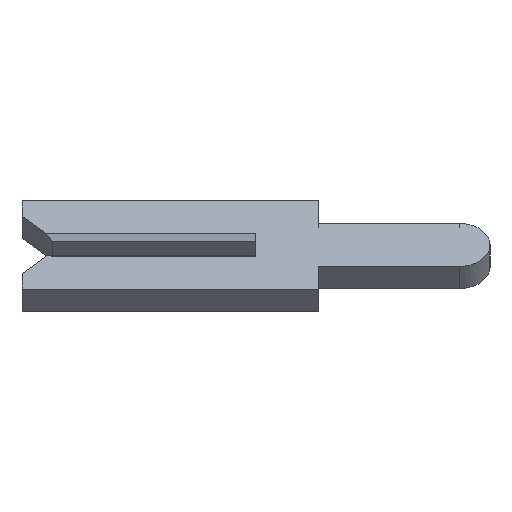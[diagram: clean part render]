
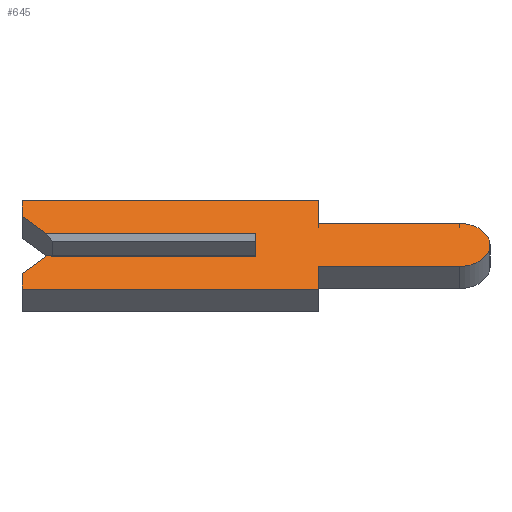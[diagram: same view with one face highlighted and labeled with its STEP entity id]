
A CAD part, left-side view. The second image highlights one B-rep face of the part: STEP entity #645.
In plain terms, the highlighted face is planar.
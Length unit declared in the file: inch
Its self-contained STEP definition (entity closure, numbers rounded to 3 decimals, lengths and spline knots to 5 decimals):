
#2 = VERTEX_POINT ( 'NONE', #682 ) ;
#9 = VERTEX_POINT ( 'NONE', #167 ) ;
#14 = VECTOR ( 'NONE', #315, 39.37008 ) ;
#22 = DIRECTION ( 'NONE',  ( 0., -1., 0. ) ) ;
#23 = ORIENTED_EDGE ( 'NONE', *, *, #552, .F. ) ;
#30 = CARTESIAN_POINT ( 'NONE',  ( -0.01, -0.04, 0.04 ) ) ;
#38 = ORIENTED_EDGE ( 'NONE', *, *, #473, .F. ) ;
#52 = CARTESIAN_POINT ( 'NONE',  ( -0.01, 0.15, -0.026 ) ) ;
#77 = FACE_OUTER_BOUND ( 'NONE', #510, .T. ) ;
#93 = EDGE_CURVE ( 'NONE', #1032, #974, #1175, .T. ) ;
#94 = LINE ( 'NONE', #275, #698 ) ;
#96 = ORIENTED_EDGE ( 'NONE', *, *, #981, .F. ) ;
#99 = EDGE_CURVE ( 'NONE', #467, #673, #94, .T. ) ;
#143 = ORIENTED_EDGE ( 'NONE', *, *, #973, .F. ) ;
#149 = VECTOR ( 'NONE', #853, 39.37008 ) ;
#152 = CARTESIAN_POINT ( 'NONE',  ( -0.01, -0.1305, 0.0195 ) ) ;
#167 = CARTESIAN_POINT ( 'NONE',  ( -0.01, 0.15, 0.04 ) ) ;
#171 = ORIENTED_EDGE ( 'NONE', *, *, #1260, .F. ) ;
#174 = DIRECTION ( 'NONE',  ( 0., 1., 0. ) ) ;
#180 = CARTESIAN_POINT ( 'NONE',  ( -0.01, 0., -0.01 ) ) ;
#188 = CARTESIAN_POINT ( 'NONE',  ( -0.01, 0.15, 0.026 ) ) ;
#198 = ORIENTED_EDGE ( 'NONE', *, *, #1116, .F. ) ;
#201 = AXIS2_PLACEMENT_3D ( 'NONE', #718, #932, #1027 ) ;
#202 = LINE ( 'NONE', #454, #268 ) ;
#247 = VERTEX_POINT ( 'NONE', #1136 ) ;
#257 = CARTESIAN_POINT ( 'NONE',  ( -0.01, 0.15, 0.01 ) ) ;
#263 = ORIENTED_EDGE ( 'NONE', *, *, #450, .F. ) ;
#266 = LINE ( 'NONE', #834, #333 ) ;
#268 = VECTOR ( 'NONE', #665, 39.37008 ) ;
#275 = CARTESIAN_POINT ( 'NONE',  ( -0.01, 0.15, -0.04 ) ) ;
#300 = CARTESIAN_POINT ( 'NONE',  ( -0.01, 0.1305, 0.0065 ) ) ;
#315 = DIRECTION ( 'NONE',  ( 0., 0., -1. ) ) ;
#329 = LINE ( 'NONE', #1117, #660 ) ;
#333 = VECTOR ( 'NONE', #733, 39.37008 ) ;
#335 = CARTESIAN_POINT ( 'NONE',  ( -0.01, 0.15, 0.04 ) ) ;
#349 = VECTOR ( 'NONE', #22, 39.37008 ) ;
#366 = CARTESIAN_POINT ( 'NONE',  ( -0.01, -0.1305, -0.0195 ) ) ;
#375 = CARTESIAN_POINT ( 'NONE',  ( -0.01, -0.1305, 0. ) ) ;
#390 = LINE ( 'NONE', #1219, #14 ) ;
#395 = CARTESIAN_POINT ( 'NONE',  ( -0.01, -0.04, -0.04 ) ) ;
#418 = LINE ( 'NONE', #335, #349 ) ;
#430 = CARTESIAN_POINT ( 'NONE',  ( -0.01, 0.134, -0.01 ) ) ;
#436 = EDGE_CURVE ( 'NONE', #823, #467, #390, .T. ) ;
#450 = EDGE_CURVE ( 'NONE', #542, #2, #329, .T. ) ;
#454 = CARTESIAN_POINT ( 'NONE',  ( -0.01, -0.1305, -0.01 ) ) ;
#467 = VERTEX_POINT ( 'NONE', #395 ) ;
#469 = DIRECTION ( 'NONE',  ( 0., 0., -1. ) ) ;
#473 = EDGE_CURVE ( 'NONE', #1114, #247, #525, .T. ) ;
#487 = VECTOR ( 'NONE', #1306, 39.37008 ) ;
#506 = VECTOR ( 'NONE', #1205, 39.37008 ) ;
#510 = EDGE_LOOP ( 'NONE', ( #558, #171, #96, #1262, #835, #723, #996, #143, #680, #23, #263, #984, #198, #38 ) ) ;
#512 = DIRECTION ( 'NONE',  ( 0., 0., -1. ) ) ;
#519 = CARTESIAN_POINT ( 'NONE',  ( -0.01, 0., 0.01 ) ) ;
#525 = LINE ( 'NONE', #300, #938 ) ;
#540 = VECTOR ( 'NONE', #1294, 39.37008 ) ;
#542 = VERTEX_POINT ( 'NONE', #30 ) ;
#552 = EDGE_CURVE ( 'NONE', #2, #1032, #266, .T. ) ;
#558 = ORIENTED_EDGE ( 'NONE', *, *, #1046, .T. ) ;
#564 = DIRECTION ( 'NONE',  ( 0., -0.707, 0.707 ) ) ;
#605 = LINE ( 'NONE', #1202, #506 ) ;
#631 = EDGE_CURVE ( 'NONE', #9, #542, #418, .T. ) ;
#645 = ADVANCED_FACE ( 'NONE', ( #77 ), #821, .F. ) ;
#659 = CARTESIAN_POINT ( 'NONE',  ( -0.01, -0.04, -0.0195 ) ) ;
#660 = VECTOR ( 'NONE', #512, 39.37008 ) ;
#665 = DIRECTION ( 'NONE',  ( 0., -1., 0. ) ) ;
#673 = VERTEX_POINT ( 'NONE', #927 ) ;
#680 = ORIENTED_EDGE ( 'NONE', *, *, #93, .F. ) ;
#682 = CARTESIAN_POINT ( 'NONE',  ( -0.01, -0.04, 0.0195 ) ) ;
#693 = VERTEX_POINT ( 'NONE', #519 ) ;
#698 = VECTOR ( 'NONE', #174, 39.37008 ) ;
#718 = CARTESIAN_POINT ( 'NONE',  ( -0.01, -0.1305, 0. ) ) ;
#723 = ORIENTED_EDGE ( 'NONE', *, *, #99, .F. ) ;
#733 = DIRECTION ( 'NONE',  ( 0., -1., 0. ) ) ;
#747 = VERTEX_POINT ( 'NONE', #430 ) ;
#774 = EDGE_CURVE ( 'NONE', #673, #1305, #1124, .T. ) ;
#779 = LINE ( 'NONE', #1276, #872 ) ;
#795 = CARTESIAN_POINT ( 'NONE',  ( -0.01, 0.15, -0.026 ) ) ;
#821 = PLANE ( 'NONE',  #201 ) ;
#823 = VERTEX_POINT ( 'NONE', #960 ) ;
#834 = CARTESIAN_POINT ( 'NONE',  ( -0.01, -0.04, 0.0195 ) ) ;
#835 = ORIENTED_EDGE ( 'NONE', *, *, #774, .F. ) ;
#853 = DIRECTION ( 'NONE',  ( 0., 0., 1. ) ) ;
#865 = DIRECTION ( 'NONE',  ( 0., -1., 0. ) ) ;
#872 = VECTOR ( 'NONE', #564, 39.37008 ) ;
#911 = LINE ( 'NONE', #659, #540 ) ;
#927 = CARTESIAN_POINT ( 'NONE',  ( -0.01, 0.15, -0.04 ) ) ;
#932 = DIRECTION ( 'NONE',  ( 1., 0., 0. ) ) ;
#938 = VECTOR ( 'NONE', #1227, 39.37008 ) ;
#947 = EDGE_CURVE ( 'NONE', #1305, #747, #779, .T. ) ;
#955 = VECTOR ( 'NONE', #865, 39.37008 ) ;
#960 = CARTESIAN_POINT ( 'NONE',  ( -0.01, -0.04, -0.0195 ) ) ;
#969 = CARTESIAN_POINT ( 'NONE',  ( -0.01, 0.134, 0.01 ) ) ;
#973 = EDGE_CURVE ( 'NONE', #974, #823, #911, .T. ) ;
#974 = VERTEX_POINT ( 'NONE', #366 ) ;
#981 = EDGE_CURVE ( 'NONE', #747, #1243, #202, .T. ) ;
#984 = ORIENTED_EDGE ( 'NONE', *, *, #631, .F. ) ;
#996 = ORIENTED_EDGE ( 'NONE', *, *, #436, .F. ) ;
#1027 = DIRECTION ( 'NONE',  ( 0., 0., -1. ) ) ;
#1032 = VERTEX_POINT ( 'NONE', #152 ) ;
#1046 = EDGE_CURVE ( 'NONE', #1114, #693, #1310, .T. ) ;
#1097 = DIRECTION ( 'NONE',  ( 1., 0., 0. ) ) ;
#1114 = VERTEX_POINT ( 'NONE', #969 ) ;
#1116 = EDGE_CURVE ( 'NONE', #247, #9, #1265, .T. ) ;
#1117 = CARTESIAN_POINT ( 'NONE',  ( -0.01, -0.04, 0.04 ) ) ;
#1124 = LINE ( 'NONE', #52, #149 ) ;
#1136 = CARTESIAN_POINT ( 'NONE',  ( -0.01, 0.15, 0.026 ) ) ;
#1175 = CIRCLE ( 'NONE', #1190, 0.0195 ) ;
#1190 = AXIS2_PLACEMENT_3D ( 'NONE', #375, #1097, #469 ) ;
#1202 = CARTESIAN_POINT ( 'NONE',  ( -0.01, 0., 0.0065 ) ) ;
#1205 = DIRECTION ( 'NONE',  ( 0., 0., 1. ) ) ;
#1219 = CARTESIAN_POINT ( 'NONE',  ( -0.01, -0.04, -0.04 ) ) ;
#1227 = DIRECTION ( 'NONE',  ( 0., 0.707, 0.707 ) ) ;
#1243 = VERTEX_POINT ( 'NONE', #180 ) ;
#1260 = EDGE_CURVE ( 'NONE', #1243, #693, #605, .T. ) ;
#1262 = ORIENTED_EDGE ( 'NONE', *, *, #947, .F. ) ;
#1265 = LINE ( 'NONE', #188, #487 ) ;
#1276 = CARTESIAN_POINT ( 'NONE',  ( -0.01, 0.1305, -0.0065 ) ) ;
#1294 = DIRECTION ( 'NONE',  ( 0., 1., 0. ) ) ;
#1305 = VERTEX_POINT ( 'NONE', #795 ) ;
#1306 = DIRECTION ( 'NONE',  ( 0., 0., 1. ) ) ;
#1310 = LINE ( 'NONE', #257, #955 ) ;
